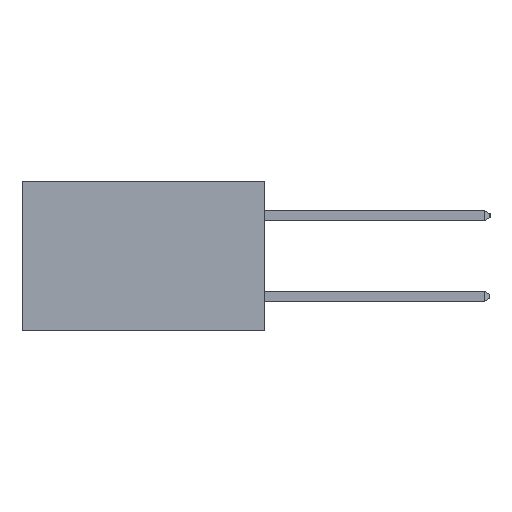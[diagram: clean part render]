
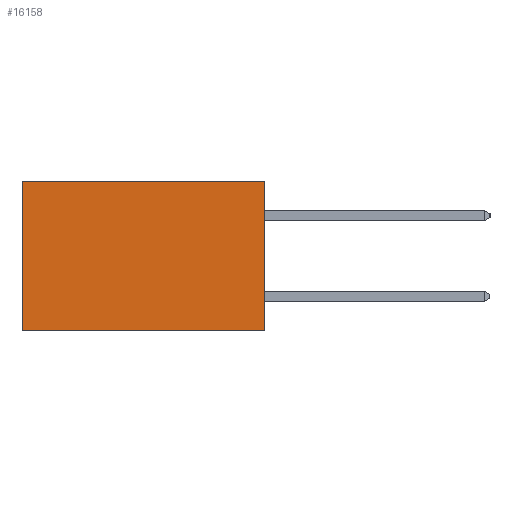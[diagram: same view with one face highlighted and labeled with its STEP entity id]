
A CAD part, left-side view. The second image highlights one B-rep face of the part: STEP entity #16158.
In plain terms, the highlighted planar face has unit normal (-1, 0, 0).
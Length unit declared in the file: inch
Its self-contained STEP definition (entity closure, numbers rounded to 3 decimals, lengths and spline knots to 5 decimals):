
#131 = CARTESIAN_POINT ( 'NONE',  ( 0.298, 0., 0. ) ) ;
#143 = LINE ( 'NONE', #18292, #17680 ) ;
#1059 = DIRECTION ( 'NONE',  ( 0., 0., -1. ) ) ;
#1522 = CARTESIAN_POINT ( 'NONE',  ( 0.298, 0., -0.37 ) ) ;
#1530 = CARTESIAN_POINT ( 'NONE',  ( 0.298, 0.6, -0.37 ) ) ;
#3860 = EDGE_CURVE ( 'NONE', #19241, #12068, #16461, .T. ) ;
#4018 = PLANE ( 'NONE',  #13203 ) ;
#4184 = LINE ( 'NONE', #14403, #21667 ) ;
#5718 = DIRECTION ( 'NONE',  ( 1., 0., 0. ) ) ;
#6119 = EDGE_CURVE ( 'NONE', #19241, #6976, #6191, .T. ) ;
#6130 = ORIENTED_EDGE ( 'NONE', *, *, #3860, .F. ) ;
#6191 = LINE ( 'NONE', #18879, #14694 ) ;
#6976 = VERTEX_POINT ( 'NONE', #21434 ) ;
#7022 = DIRECTION ( 'NONE',  ( 0., 1., 0. ) ) ;
#7960 = ORIENTED_EDGE ( 'NONE', *, *, #16502, .T. ) ;
#8573 = ORIENTED_EDGE ( 'NONE', *, *, #6119, .T. ) ;
#8761 = ORIENTED_EDGE ( 'NONE', *, *, #15415, .F. ) ;
#9804 = DIRECTION ( 'NONE',  ( 0., 0., -1. ) ) ;
#10666 = CARTESIAN_POINT ( 'NONE',  ( 0.298, 0., 0. ) ) ;
#10735 = FACE_OUTER_BOUND ( 'NONE', #12991, .T. ) ;
#12068 = VERTEX_POINT ( 'NONE', #1522 ) ;
#12991 = EDGE_LOOP ( 'NONE', ( #7960, #8761, #6130, #8573 ) ) ;
#13203 = AXIS2_PLACEMENT_3D ( 'NONE', #15876, #5718, #17562 ) ;
#14403 = CARTESIAN_POINT ( 'NONE',  ( 0.298, 0., -0.37 ) ) ;
#14694 = VECTOR ( 'NONE', #7022, 39.37008 ) ;
#15415 = EDGE_CURVE ( 'NONE', #12068, #16573, #4184, .T. ) ;
#15876 = CARTESIAN_POINT ( 'NONE',  ( 0.298, 0., 0. ) ) ;
#16114 = DIRECTION ( 'NONE',  ( 0., 1., 0. ) ) ;
#16158 = ADVANCED_FACE ( 'NONE', ( #10735 ), #4018, .F. ) ;
#16461 = LINE ( 'NONE', #131, #20444 ) ;
#16502 = EDGE_CURVE ( 'NONE', #6976, #16573, #143, .T. ) ;
#16573 = VERTEX_POINT ( 'NONE', #1530 ) ;
#17562 = DIRECTION ( 'NONE',  ( 0., 0., -1. ) ) ;
#17680 = VECTOR ( 'NONE', #9804, 39.37008 ) ;
#18292 = CARTESIAN_POINT ( 'NONE',  ( 0.298, 0.6, 0. ) ) ;
#18879 = CARTESIAN_POINT ( 'NONE',  ( 0.298, 0., 0. ) ) ;
#19241 = VERTEX_POINT ( 'NONE', #10666 ) ;
#20444 = VECTOR ( 'NONE', #1059, 39.37008 ) ;
#21434 = CARTESIAN_POINT ( 'NONE',  ( 0.298, 0.6, 0. ) ) ;
#21667 = VECTOR ( 'NONE', #16114, 39.37008 ) ;
